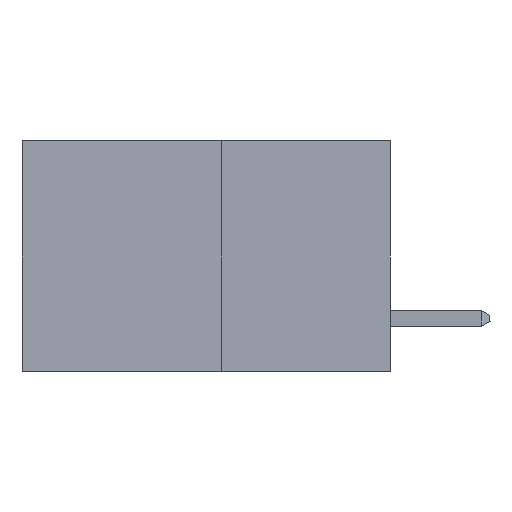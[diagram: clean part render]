
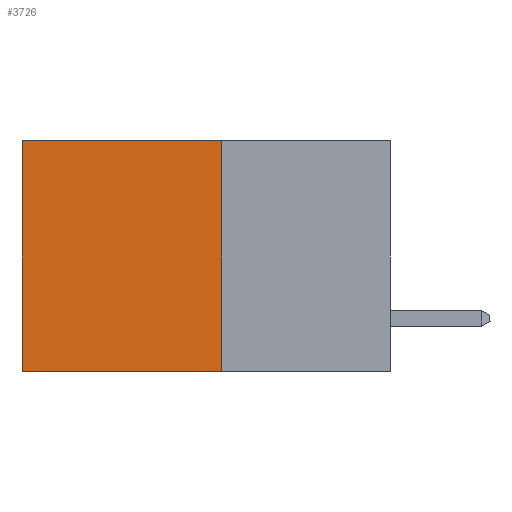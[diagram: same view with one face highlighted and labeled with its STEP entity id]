
A CAD part, left-side view. The second image highlights one B-rep face of the part: STEP entity #3726.
In plain terms, the highlighted planar face has unit normal (-1, 0, 0).
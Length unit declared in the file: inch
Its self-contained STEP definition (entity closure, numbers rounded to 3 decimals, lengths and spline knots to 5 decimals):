
#275 = EDGE_CURVE ( 'NONE', #5693, #4415, #683, .T. ) ;
#345 = VECTOR ( 'NONE', #406, 39.37008 ) ;
#406 = DIRECTION ( 'NONE',  ( 0., 1., 0. ) ) ;
#683 = LINE ( 'NONE', #7162, #10067 ) ;
#706 = AXIS2_PLACEMENT_3D ( 'NONE', #4026, #10373, #10350 ) ;
#831 = ORIENTED_EDGE ( 'NONE', *, *, #8484, .T. ) ;
#964 = CARTESIAN_POINT ( 'NONE',  ( 0.277, 0.27, 0. ) ) ;
#1181 = DIRECTION ( 'NONE',  ( 0., 0., -1. ) ) ;
#1309 = EDGE_CURVE ( 'NONE', #4415, #3426, #5300, .T. ) ;
#1840 = CARTESIAN_POINT ( 'NONE',  ( 0.277, 0.27, 0. ) ) ;
#2055 = VERTEX_POINT ( 'NONE', #7197 ) ;
#3198 = EDGE_LOOP ( 'NONE', ( #10823, #5580, #10841, #831 ) ) ;
#3426 = VERTEX_POINT ( 'NONE', #7267 ) ;
#3726 = ADVANCED_FACE ( 'NONE', ( #5661 ), #7938, .F. ) ;
#4026 = CARTESIAN_POINT ( 'NONE',  ( 0.277, 0.27, -0.37 ) ) ;
#4078 = CARTESIAN_POINT ( 'NONE',  ( 0.277, 0.59, -0.37 ) ) ;
#4415 = VERTEX_POINT ( 'NONE', #8442 ) ;
#5300 = LINE ( 'NONE', #10630, #345 ) ;
#5580 = ORIENTED_EDGE ( 'NONE', *, *, #1309, .F. ) ;
#5661 = FACE_OUTER_BOUND ( 'NONE', #3198, .T. ) ;
#5693 = VERTEX_POINT ( 'NONE', #1840 ) ;
#5778 = EDGE_CURVE ( 'NONE', #2055, #3426, #11606, .T. ) ;
#6237 = LINE ( 'NONE', #964, #10341 ) ;
#7162 = CARTESIAN_POINT ( 'NONE',  ( 0.277, 0.27, -0.37 ) ) ;
#7197 = CARTESIAN_POINT ( 'NONE',  ( 0.277, 0.59, 0. ) ) ;
#7267 = CARTESIAN_POINT ( 'NONE',  ( 0.277, 0.59, -0.37 ) ) ;
#7938 = PLANE ( 'NONE',  #706 ) ;
#8442 = CARTESIAN_POINT ( 'NONE',  ( 0.277, 0.27, -0.37 ) ) ;
#8484 = EDGE_CURVE ( 'NONE', #5693, #2055, #6237, .T. ) ;
#9137 = DIRECTION ( 'NONE',  ( 0., 1., 0. ) ) ;
#9556 = VECTOR ( 'NONE', #10035, 39.37008 ) ;
#10035 = DIRECTION ( 'NONE',  ( 0., 0., -1. ) ) ;
#10067 = VECTOR ( 'NONE', #1181, 39.37008 ) ;
#10341 = VECTOR ( 'NONE', #9137, 39.37008 ) ;
#10350 = DIRECTION ( 'NONE',  ( 0., 0., -1. ) ) ;
#10373 = DIRECTION ( 'NONE',  ( 1., 0., 0. ) ) ;
#10630 = CARTESIAN_POINT ( 'NONE',  ( 0.277, 0.27, -0.37 ) ) ;
#10823 = ORIENTED_EDGE ( 'NONE', *, *, #5778, .T. ) ;
#10841 = ORIENTED_EDGE ( 'NONE', *, *, #275, .F. ) ;
#11606 = LINE ( 'NONE', #4078, #9556 ) ;
